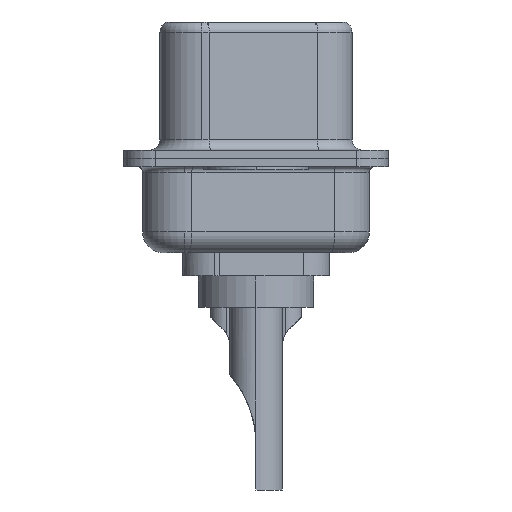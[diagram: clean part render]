
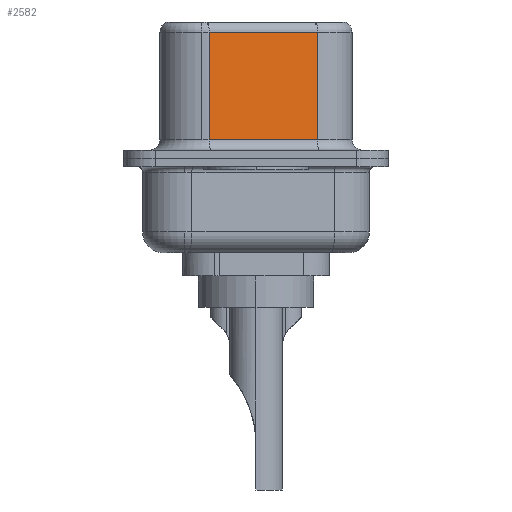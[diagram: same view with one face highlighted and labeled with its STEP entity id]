
A CAD part, left-side view. The second image highlights one B-rep face of the part: STEP entity #2582.
In plain terms, the highlighted planar face has unit normal (-0.985, -0.174, 0).
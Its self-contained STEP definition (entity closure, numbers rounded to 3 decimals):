
#329 = CARTESIAN_POINT ( 'NONE',  ( 4.58, -2.927, 0.9 ) ) ;
#1094 = VECTOR ( 'NONE', #9735, 1000. ) ;
#1327 = VECTOR ( 'NONE', #3928, 1000. ) ;
#1572 = LINE ( 'NONE', #10450, #9447 ) ;
#1702 = VERTEX_POINT ( 'NONE', #9545 ) ;
#1835 = LINE ( 'NONE', #13264, #1327 ) ;
#2097 = AXIS2_PLACEMENT_3D ( 'NONE', #3793, #6769, #12852 ) ;
#2272 = VERTEX_POINT ( 'NONE', #14694 ) ;
#2582 = ADVANCED_FACE ( 'NONE', ( #15790 ), #6863, .F. ) ;
#3721 = CARTESIAN_POINT ( 'NONE',  ( 4.58, -2.927, 6.02 ) ) ;
#3793 = CARTESIAN_POINT ( 'NONE',  ( 4.58, -2.927, 6.52 ) ) ;
#3928 = DIRECTION ( 'NONE',  ( -0.174, 0.985, 0. ) ) ;
#4772 = EDGE_LOOP ( 'NONE', ( #12018, #10363, #14844, #4906 ) ) ;
#4906 = ORIENTED_EDGE ( 'NONE', *, *, #8462, .T. ) ;
#5239 = LINE ( 'NONE', #17198, #1094 ) ;
#6769 = DIRECTION ( 'NONE',  ( 0.985, 0.174, 0. ) ) ;
#6863 = PLANE ( 'NONE',  #2097 ) ;
#7312 = VERTEX_POINT ( 'NONE', #329 ) ;
#8462 = EDGE_CURVE ( 'NONE', #1702, #7312, #5239, .T. ) ;
#9447 = VECTOR ( 'NONE', #9774, 1000. ) ;
#9545 = CARTESIAN_POINT ( 'NONE',  ( 3.67, 2.233, 0.9 ) ) ;
#9557 = EDGE_CURVE ( 'NONE', #12465, #7312, #1572, .T. ) ;
#9735 = DIRECTION ( 'NONE',  ( 0.174, -0.985, 0. ) ) ;
#9774 = DIRECTION ( 'NONE',  ( 0., 0., -1. ) ) ;
#10363 = ORIENTED_EDGE ( 'NONE', *, *, #15044, .T. ) ;
#10450 = CARTESIAN_POINT ( 'NONE',  ( 4.58, -2.927, 6.52 ) ) ;
#10837 = CARTESIAN_POINT ( 'NONE',  ( 3.67, 2.233, 6.52 ) ) ;
#12018 = ORIENTED_EDGE ( 'NONE', *, *, #9557, .F. ) ;
#12332 = DIRECTION ( 'NONE',  ( 0., 0., -1. ) ) ;
#12465 = VERTEX_POINT ( 'NONE', #3721 ) ;
#12852 = DIRECTION ( 'NONE',  ( -0.174, 0.985, 0. ) ) ;
#13264 = CARTESIAN_POINT ( 'NONE',  ( 4.58, -2.927, 6.02 ) ) ;
#14694 = CARTESIAN_POINT ( 'NONE',  ( 3.67, 2.233, 6.02 ) ) ;
#14844 = ORIENTED_EDGE ( 'NONE', *, *, #19807, .T. ) ;
#15044 = EDGE_CURVE ( 'NONE', #12465, #2272, #1835, .T. ) ;
#15790 = FACE_OUTER_BOUND ( 'NONE', #4772, .T. ) ;
#16430 = VECTOR ( 'NONE', #12332, 1000. ) ;
#16882 = LINE ( 'NONE', #10837, #16430 ) ;
#17198 = CARTESIAN_POINT ( 'NONE',  ( 4.58, -2.927, 0.9 ) ) ;
#19807 = EDGE_CURVE ( 'NONE', #2272, #1702, #16882, .T. ) ;
